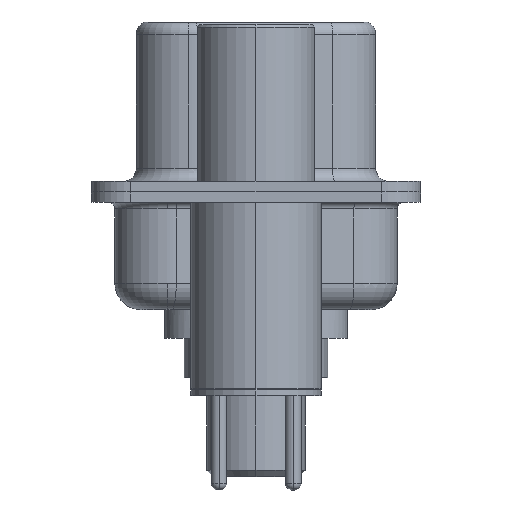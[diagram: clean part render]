
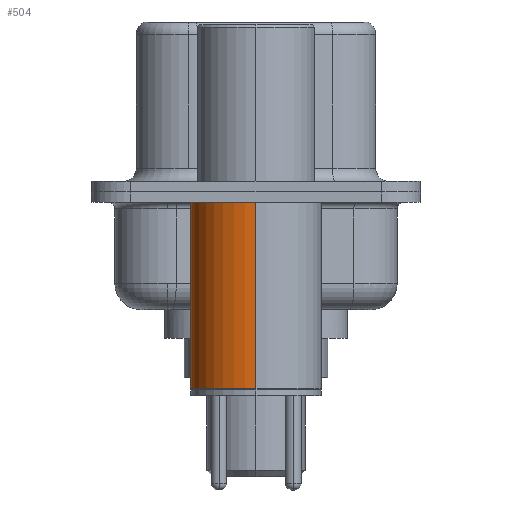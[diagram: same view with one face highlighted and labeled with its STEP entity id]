
A CAD part, left-side view. The second image highlights one B-rep face of the part: STEP entity #504.
In plain terms, the highlighted cylindrical face has radius 2.5 mm (diameter 5 mm), a partial arc.
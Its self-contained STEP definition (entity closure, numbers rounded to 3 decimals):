
#504 = ADVANCED_FACE ( 'NONE', ( #13267 ), #12670, .T. ) ;
#782 = DIRECTION ( 'NONE',  ( 0., 0., 1. ) ) ;
#1144 = DIRECTION ( 'NONE',  ( 0., 0., 1. ) ) ;
#1276 = EDGE_CURVE ( 'NONE', #23874, #16192, #15267, .T. ) ;
#1409 = DIRECTION ( 'NONE',  ( 0., 0., 1. ) ) ;
#1927 = CARTESIAN_POINT ( 'NONE',  ( -2.5, 0., -7.525 ) ) ;
#2935 = CARTESIAN_POINT ( 'NONE',  ( 2.5, 0., -0.4 ) ) ;
#3454 = LINE ( 'NONE', #17061, #22674 ) ;
#3914 = DIRECTION ( 'NONE',  ( 0., 0., 1. ) ) ;
#4495 = CARTESIAN_POINT ( 'NONE',  ( -2.5, 0., -0.4 ) ) ;
#4640 = DIRECTION ( 'NONE',  ( 0., 0., 1. ) ) ;
#5069 = EDGE_CURVE ( 'NONE', #19750, #16192, #3454, .T. ) ;
#5450 = VECTOR ( 'NONE', #3914, 1000. ) ;
#5878 = CARTESIAN_POINT ( 'NONE',  ( 2.5, 0., 0.581 ) ) ;
#6324 = EDGE_CURVE ( 'NONE', #19841, #19750, #21659, .T. ) ;
#6394 = CARTESIAN_POINT ( 'NONE',  ( 0., 0., 0.581 ) ) ;
#7348 = AXIS2_PLACEMENT_3D ( 'NONE', #12358, #1144, #14192 ) ;
#8518 = AXIS2_PLACEMENT_3D ( 'NONE', #20903, #4640, #18277 ) ;
#9497 = ORIENTED_EDGE ( 'NONE', *, *, #24185, .F. ) ;
#12358 = CARTESIAN_POINT ( 'NONE',  ( 0., 0., -7.525 ) ) ;
#12670 = CYLINDRICAL_SURFACE ( 'NONE', #13652, 2.5 ) ;
#13267 = FACE_OUTER_BOUND ( 'NONE', #18843, .T. ) ;
#13652 = AXIS2_PLACEMENT_3D ( 'NONE', #6394, #1409, #15896 ) ;
#14192 = DIRECTION ( 'NONE',  ( 1., 0., 0. ) ) ;
#15267 = CIRCLE ( 'NONE', #8518, 2.5 ) ;
#15896 = DIRECTION ( 'NONE',  ( 1., 0., 0. ) ) ;
#16192 = VERTEX_POINT ( 'NONE', #4495 ) ;
#17061 = CARTESIAN_POINT ( 'NONE',  ( -2.5, 0., 0.581 ) ) ;
#17939 = ORIENTED_EDGE ( 'NONE', *, *, #1276, .F. ) ;
#18277 = DIRECTION ( 'NONE',  ( 1., 0., 0. ) ) ;
#18843 = EDGE_LOOP ( 'NONE', ( #20165, #22579, #17939, #9497 ) ) ;
#18854 = CARTESIAN_POINT ( 'NONE',  ( 2.5, 0., -7.525 ) ) ;
#19750 = VERTEX_POINT ( 'NONE', #1927 ) ;
#19841 = VERTEX_POINT ( 'NONE', #18854 ) ;
#20165 = ORIENTED_EDGE ( 'NONE', *, *, #6324, .T. ) ;
#20874 = LINE ( 'NONE', #5878, #5450 ) ;
#20903 = CARTESIAN_POINT ( 'NONE',  ( 0., 0., -0.4 ) ) ;
#21659 = CIRCLE ( 'NONE', #7348, 2.5 ) ;
#22579 = ORIENTED_EDGE ( 'NONE', *, *, #5069, .T. ) ;
#22674 = VECTOR ( 'NONE', #782, 1000. ) ;
#23874 = VERTEX_POINT ( 'NONE', #2935 ) ;
#24185 = EDGE_CURVE ( 'NONE', #19841, #23874, #20874, .T. ) ;
